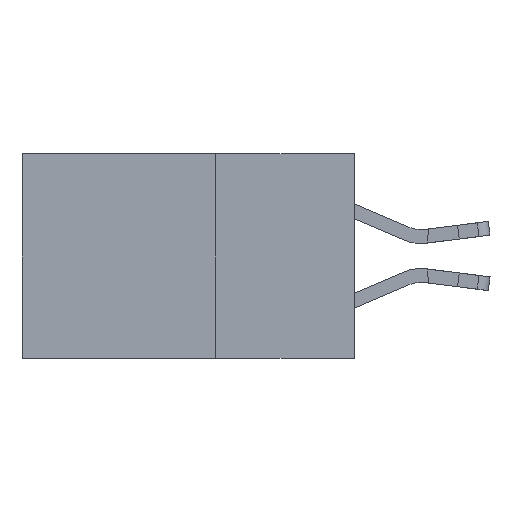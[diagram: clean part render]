
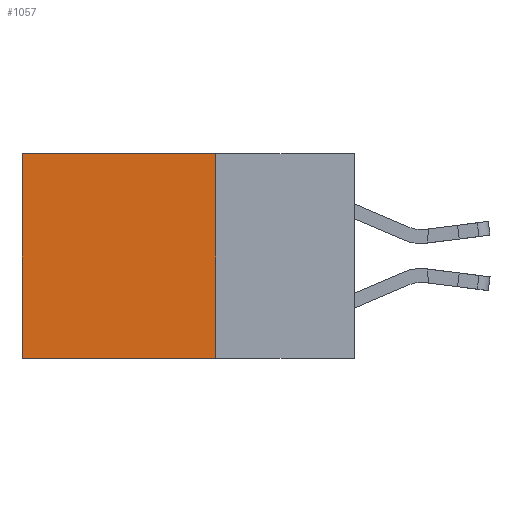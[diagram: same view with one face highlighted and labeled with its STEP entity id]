
A CAD part, left-side view. The second image highlights one B-rep face of the part: STEP entity #1057.
In plain terms, the highlighted planar face has unit normal (-1, 0, 0).
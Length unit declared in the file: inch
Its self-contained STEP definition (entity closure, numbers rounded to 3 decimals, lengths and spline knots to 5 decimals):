
#4 = CARTESIAN_POINT ( 'NONE',  ( 0.2615, 0.25, 0. ) ) ;
#521 = LINE ( 'NONE', #6012, #3647 ) ;
#698 = VECTOR ( 'NONE', #3997, 39.37008 ) ;
#981 = ORIENTED_EDGE ( 'NONE', *, *, #9544, .T. ) ;
#1057 = ADVANCED_FACE ( 'NONE', ( #2346 ), #7494, .F. ) ;
#1619 = VECTOR ( 'NONE', #15069, 39.37008 ) ;
#2346 = FACE_OUTER_BOUND ( 'NONE', #14534, .T. ) ;
#3439 = ORIENTED_EDGE ( 'NONE', *, *, #11285, .T. ) ;
#3647 = VECTOR ( 'NONE', #6144, 39.37008 ) ;
#3997 = DIRECTION ( 'NONE',  ( 0., 0., -1. ) ) ;
#4145 = CARTESIAN_POINT ( 'NONE',  ( 0.2615, 0.25, -0.37 ) ) ;
#4527 = VERTEX_POINT ( 'NONE', #12155 ) ;
#4882 = VECTOR ( 'NONE', #11213, 39.37008 ) ;
#5116 = LINE ( 'NONE', #4, #1619 ) ;
#5269 = LINE ( 'NONE', #10932, #4882 ) ;
#6012 = CARTESIAN_POINT ( 'NONE',  ( 0.2615, 0.6, -0.37 ) ) ;
#6144 = DIRECTION ( 'NONE',  ( 0., 0., -1. ) ) ;
#6759 = ORIENTED_EDGE ( 'NONE', *, *, #12758, .F. ) ;
#7494 = PLANE ( 'NONE',  #13646 ) ;
#7614 = VERTEX_POINT ( 'NONE', #7865 ) ;
#7865 = CARTESIAN_POINT ( 'NONE',  ( 0.2615, 0.6, -0.37 ) ) ;
#8143 = CARTESIAN_POINT ( 'NONE',  ( 0.2615, 0.25, 0. ) ) ;
#9544 = EDGE_CURVE ( 'NONE', #14174, #4527, #5116, .T. ) ;
#9584 = VERTEX_POINT ( 'NONE', #13445 ) ;
#10262 = EDGE_CURVE ( 'NONE', #9584, #7614, #5269, .T. ) ;
#10341 = DIRECTION ( 'NONE',  ( 1., 0., 0. ) ) ;
#10346 = DIRECTION ( 'NONE',  ( 0., 0., -1. ) ) ;
#10517 = CARTESIAN_POINT ( 'NONE',  ( 0.2615, 0.25, -0.37 ) ) ;
#10923 = LINE ( 'NONE', #4145, #698 ) ;
#10932 = CARTESIAN_POINT ( 'NONE',  ( 0.2615, 0.25, -0.37 ) ) ;
#11213 = DIRECTION ( 'NONE',  ( 0., 1., 0. ) ) ;
#11285 = EDGE_CURVE ( 'NONE', #4527, #7614, #521, .T. ) ;
#12155 = CARTESIAN_POINT ( 'NONE',  ( 0.2615, 0.6, 0. ) ) ;
#12758 = EDGE_CURVE ( 'NONE', #14174, #9584, #10923, .T. ) ;
#13445 = CARTESIAN_POINT ( 'NONE',  ( 0.2615, 0.25, -0.37 ) ) ;
#13646 = AXIS2_PLACEMENT_3D ( 'NONE', #10517, #10341, #10346 ) ;
#14174 = VERTEX_POINT ( 'NONE', #8143 ) ;
#14240 = ORIENTED_EDGE ( 'NONE', *, *, #10262, .F. ) ;
#14534 = EDGE_LOOP ( 'NONE', ( #3439, #14240, #6759, #981 ) ) ;
#15069 = DIRECTION ( 'NONE',  ( 0., 1., 0. ) ) ;
